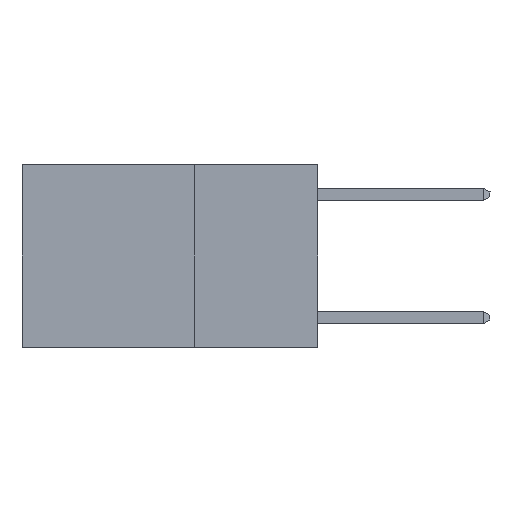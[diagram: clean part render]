
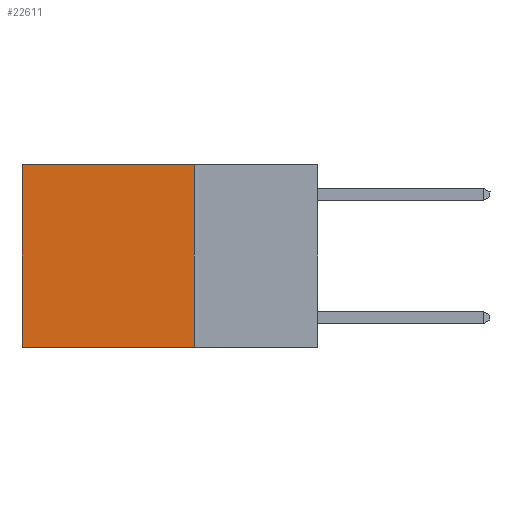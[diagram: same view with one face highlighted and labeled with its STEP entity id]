
A CAD part, left-side view. The second image highlights one B-rep face of the part: STEP entity #22611.
In plain terms, the highlighted planar face has unit normal (-1, 0, 0).
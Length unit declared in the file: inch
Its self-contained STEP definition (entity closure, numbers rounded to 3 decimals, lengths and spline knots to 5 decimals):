
#803 = VERTEX_POINT ( 'NONE', #18535 ) ;
#1644 = VECTOR ( 'NONE', #8376, 39.37008 ) ;
#2529 = CARTESIAN_POINT ( 'NONE',  ( 0.2625, 0.6, 0. ) ) ;
#4471 = PLANE ( 'NONE',  #16430 ) ;
#4861 = CARTESIAN_POINT ( 'NONE',  ( 0.2625, 0.25, -0.37 ) ) ;
#5244 = CARTESIAN_POINT ( 'NONE',  ( 0.2625, 0.6, 0. ) ) ;
#5500 = VERTEX_POINT ( 'NONE', #8845 ) ;
#5814 = EDGE_CURVE ( 'NONE', #803, #5500, #20253, .T. ) ;
#6049 = VECTOR ( 'NONE', #15169, 39.37008 ) ;
#6303 = DIRECTION ( 'NONE',  ( 0., 0., -1. ) ) ;
#6537 = EDGE_CURVE ( 'NONE', #5500, #21319, #19948, .T. ) ;
#7131 = FACE_OUTER_BOUND ( 'NONE', #21674, .T. ) ;
#7264 = EDGE_CURVE ( 'NONE', #8283, #21319, #10332, .T. ) ;
#8283 = VERTEX_POINT ( 'NONE', #5244 ) ;
#8311 = CARTESIAN_POINT ( 'NONE',  ( 0.2625, 0.25, 0. ) ) ;
#8376 = DIRECTION ( 'NONE',  ( 0., 0., -1. ) ) ;
#8845 = CARTESIAN_POINT ( 'NONE',  ( 0.2625, 0.25, -0.37 ) ) ;
#10332 = LINE ( 'NONE', #2529, #6049 ) ;
#10442 = ORIENTED_EDGE ( 'NONE', *, *, #5814, .F. ) ;
#11895 = CARTESIAN_POINT ( 'NONE',  ( 0.2625, 0.6, -0.37 ) ) ;
#12890 = EDGE_CURVE ( 'NONE', #803, #8283, #16421, .T. ) ;
#13509 = CARTESIAN_POINT ( 'NONE',  ( 0.2625, 0.25, 0. ) ) ;
#14018 = ORIENTED_EDGE ( 'NONE', *, *, #12890, .T. ) ;
#15169 = DIRECTION ( 'NONE',  ( 0., 0., -1. ) ) ;
#16280 = VECTOR ( 'NONE', #19318, 39.37008 ) ;
#16421 = LINE ( 'NONE', #8311, #20087 ) ;
#16430 = AXIS2_PLACEMENT_3D ( 'NONE', #13509, #17120, #6303 ) ;
#17120 = DIRECTION ( 'NONE',  ( 1., 0., 0. ) ) ;
#17315 = DIRECTION ( 'NONE',  ( 0., 1., 0. ) ) ;
#18535 = CARTESIAN_POINT ( 'NONE',  ( 0.2625, 0.25, 0. ) ) ;
#19112 = CARTESIAN_POINT ( 'NONE',  ( 0.2625, 0.25, 0. ) ) ;
#19318 = DIRECTION ( 'NONE',  ( 0., 1., 0. ) ) ;
#19948 = LINE ( 'NONE', #4861, #16280 ) ;
#20087 = VECTOR ( 'NONE', #17315, 39.37008 ) ;
#20253 = LINE ( 'NONE', #19112, #1644 ) ;
#21319 = VERTEX_POINT ( 'NONE', #11895 ) ;
#21674 = EDGE_LOOP ( 'NONE', ( #22838, #22455, #10442, #14018 ) ) ;
#22455 = ORIENTED_EDGE ( 'NONE', *, *, #6537, .F. ) ;
#22611 = ADVANCED_FACE ( 'NONE', ( #7131 ), #4471, .F. ) ;
#22838 = ORIENTED_EDGE ( 'NONE', *, *, #7264, .T. ) ;
